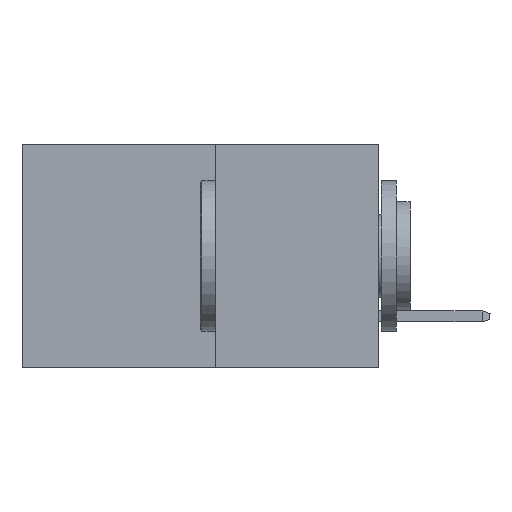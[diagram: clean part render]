
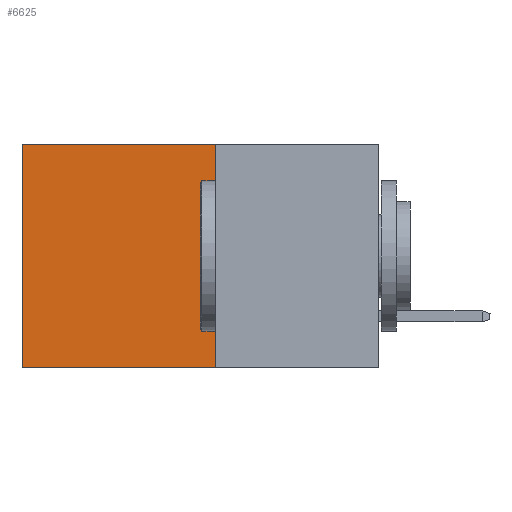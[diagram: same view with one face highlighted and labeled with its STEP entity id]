
A CAD part, left-side view. The second image highlights one B-rep face of the part: STEP entity #6625.
In plain terms, the highlighted planar face has unit normal (-1, 0, 0).
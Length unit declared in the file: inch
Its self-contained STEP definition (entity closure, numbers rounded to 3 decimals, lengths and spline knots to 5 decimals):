
#613 = DIRECTION ( 'NONE',  ( 0., 1., 0. ) ) ;
#686 = CARTESIAN_POINT ( 'NONE',  ( 0.277, 0.27, 0. ) ) ;
#990 = DIRECTION ( 'NONE',  ( 0., 1., 0. ) ) ;
#2232 = EDGE_CURVE ( 'NONE', #12751, #4621, #24110, .T. ) ;
#2623 = DIRECTION ( 'NONE',  ( 1., 0., 0. ) ) ;
#3203 = LINE ( 'NONE', #26245, #25032 ) ;
#3669 = CARTESIAN_POINT ( 'NONE',  ( 0.277, 0.27, -0.37 ) ) ;
#4358 = AXIS2_PLACEMENT_3D ( 'NONE', #15371, #2623, #17507 ) ;
#4621 = VERTEX_POINT ( 'NONE', #22817 ) ;
#6625 = ADVANCED_FACE ( 'NONE', ( #16696 ), #11077, .F. ) ;
#7335 = DIRECTION ( 'NONE',  ( 0., 0., -1. ) ) ;
#7382 = VERTEX_POINT ( 'NONE', #686 ) ;
#8102 = EDGE_CURVE ( 'NONE', #24605, #4621, #3203, .T. ) ;
#10805 = EDGE_LOOP ( 'NONE', ( #25484, #17723, #22694, #12210 ) ) ;
#11077 = PLANE ( 'NONE',  #4358 ) ;
#11152 = CARTESIAN_POINT ( 'NONE',  ( 0.277, 0.27, 0. ) ) ;
#12210 = ORIENTED_EDGE ( 'NONE', *, *, #21058, .T. ) ;
#12751 = VERTEX_POINT ( 'NONE', #16344 ) ;
#13222 = LINE ( 'NONE', #11152, #24392 ) ;
#15371 = CARTESIAN_POINT ( 'NONE',  ( 0.277, 0.27, -0.37 ) ) ;
#15407 = LINE ( 'NONE', #24223, #25203 ) ;
#16344 = CARTESIAN_POINT ( 'NONE',  ( 0.277, 0.59, 0. ) ) ;
#16696 = FACE_OUTER_BOUND ( 'NONE', #10805, .T. ) ;
#16821 = CARTESIAN_POINT ( 'NONE',  ( 0.277, 0.59, -0.37 ) ) ;
#17507 = DIRECTION ( 'NONE',  ( 0., 0., -1. ) ) ;
#17723 = ORIENTED_EDGE ( 'NONE', *, *, #8102, .F. ) ;
#18559 = VECTOR ( 'NONE', #23335, 39.37008 ) ;
#21058 = EDGE_CURVE ( 'NONE', #7382, #12751, #13222, .T. ) ;
#22694 = ORIENTED_EDGE ( 'NONE', *, *, #24413, .F. ) ;
#22817 = CARTESIAN_POINT ( 'NONE',  ( 0.277, 0.59, -0.37 ) ) ;
#23335 = DIRECTION ( 'NONE',  ( 0., 0., -1. ) ) ;
#24110 = LINE ( 'NONE', #16821, #18559 ) ;
#24223 = CARTESIAN_POINT ( 'NONE',  ( 0.277, 0.27, -0.37 ) ) ;
#24392 = VECTOR ( 'NONE', #613, 39.37008 ) ;
#24413 = EDGE_CURVE ( 'NONE', #7382, #24605, #15407, .T. ) ;
#24605 = VERTEX_POINT ( 'NONE', #3669 ) ;
#25032 = VECTOR ( 'NONE', #990, 39.37008 ) ;
#25203 = VECTOR ( 'NONE', #7335, 39.37008 ) ;
#25484 = ORIENTED_EDGE ( 'NONE', *, *, #2232, .T. ) ;
#26245 = CARTESIAN_POINT ( 'NONE',  ( 0.277, 0.27, -0.37 ) ) ;
